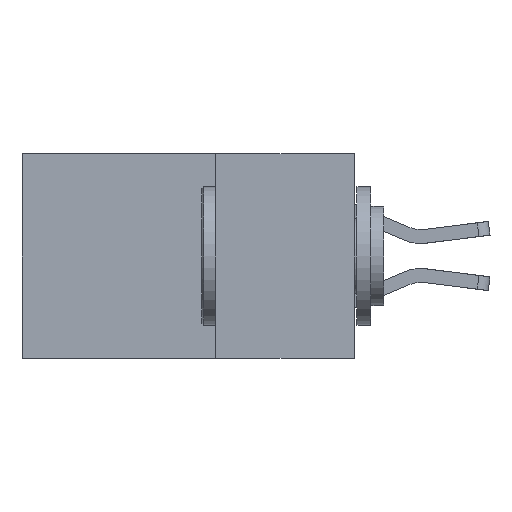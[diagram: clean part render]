
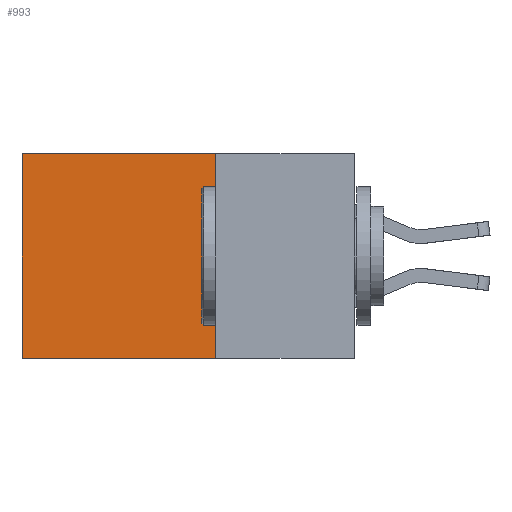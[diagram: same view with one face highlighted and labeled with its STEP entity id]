
A CAD part, left-side view. The second image highlights one B-rep face of the part: STEP entity #993.
In plain terms, the highlighted planar face has unit normal (-1, 0, 0).
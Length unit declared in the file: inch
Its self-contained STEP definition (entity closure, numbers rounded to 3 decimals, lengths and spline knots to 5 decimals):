
#119 = VECTOR ( 'NONE', #1381, 39.37008 ) ;
#214 = CARTESIAN_POINT ( 'NONE',  ( 0.2615, 0.25, -0.37 ) ) ;
#430 = EDGE_LOOP ( 'NONE', ( #1436, #7370, #1698, #3732 ) ) ;
#522 = CARTESIAN_POINT ( 'NONE',  ( 0.2615, 0.25, -0.37 ) ) ;
#621 = CARTESIAN_POINT ( 'NONE',  ( 0.2615, 0.6, -0.37 ) ) ;
#639 = VECTOR ( 'NONE', #8106, 39.37008 ) ;
#777 = PLANE ( 'NONE',  #3311 ) ;
#993 = ADVANCED_FACE ( 'NONE', ( #1563 ), #777, .F. ) ;
#1003 = DIRECTION ( 'NONE',  ( 0., 0., -1. ) ) ;
#1023 = DIRECTION ( 'NONE',  ( 1., 0., 0. ) ) ;
#1180 = CARTESIAN_POINT ( 'NONE',  ( 0.2615, 0.25, -0.37 ) ) ;
#1203 = DIRECTION ( 'NONE',  ( 0., 0., -1. ) ) ;
#1381 = DIRECTION ( 'NONE',  ( 0., 0., -1. ) ) ;
#1436 = ORIENTED_EDGE ( 'NONE', *, *, #4638, .T. ) ;
#1563 = FACE_OUTER_BOUND ( 'NONE', #430, .T. ) ;
#1698 = ORIENTED_EDGE ( 'NONE', *, *, #7174, .F. ) ;
#1836 = VERTEX_POINT ( 'NONE', #522 ) ;
#2205 = CARTESIAN_POINT ( 'NONE',  ( 0.2615, 0.25, 0. ) ) ;
#2548 = LINE ( 'NONE', #3187, #9467 ) ;
#3183 = VERTEX_POINT ( 'NONE', #5836 ) ;
#3187 = CARTESIAN_POINT ( 'NONE',  ( 0.2615, 0.25, -0.37 ) ) ;
#3311 = AXIS2_PLACEMENT_3D ( 'NONE', #1180, #1023, #1203 ) ;
#3732 = ORIENTED_EDGE ( 'NONE', *, *, #4154, .T. ) ;
#3925 = DIRECTION ( 'NONE',  ( 0., 1., 0. ) ) ;
#4044 = CARTESIAN_POINT ( 'NONE',  ( 0.2615, 0.6, -0.37 ) ) ;
#4154 = EDGE_CURVE ( 'NONE', #6989, #3183, #8340, .T. ) ;
#4638 = EDGE_CURVE ( 'NONE', #3183, #8201, #6119, .T. ) ;
#4725 = VECTOR ( 'NONE', #1003, 39.37008 ) ;
#5836 = CARTESIAN_POINT ( 'NONE',  ( 0.2615, 0.6, 0. ) ) ;
#6119 = LINE ( 'NONE', #621, #119 ) ;
#6989 = VERTEX_POINT ( 'NONE', #8817 ) ;
#7174 = EDGE_CURVE ( 'NONE', #6989, #1836, #8591, .T. ) ;
#7370 = ORIENTED_EDGE ( 'NONE', *, *, #7580, .F. ) ;
#7580 = EDGE_CURVE ( 'NONE', #1836, #8201, #2548, .T. ) ;
#8106 = DIRECTION ( 'NONE',  ( 0., 1., 0. ) ) ;
#8201 = VERTEX_POINT ( 'NONE', #4044 ) ;
#8340 = LINE ( 'NONE', #2205, #639 ) ;
#8591 = LINE ( 'NONE', #214, #4725 ) ;
#8817 = CARTESIAN_POINT ( 'NONE',  ( 0.2615, 0.25, 0. ) ) ;
#9467 = VECTOR ( 'NONE', #3925, 39.37008 ) ;
